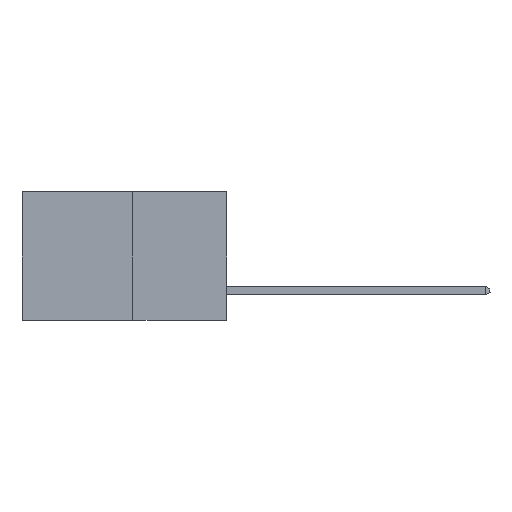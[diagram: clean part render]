
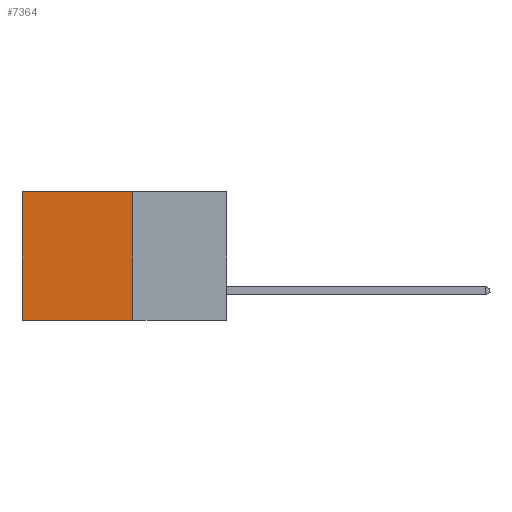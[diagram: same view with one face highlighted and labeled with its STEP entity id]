
A CAD part, left-side view. The second image highlights one B-rep face of the part: STEP entity #7364.
In plain terms, the highlighted planar face has unit normal (-1, 0, 0).
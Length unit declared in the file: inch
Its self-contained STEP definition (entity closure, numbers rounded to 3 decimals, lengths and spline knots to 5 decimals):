
#1385 = LINE ( 'NONE', #20983, #14818 ) ;
#3186 = CARTESIAN_POINT ( 'NONE',  ( 0.277, 0.59, -0.37 ) ) ;
#3329 = CARTESIAN_POINT ( 'NONE',  ( 0.277, 0.59, 0. ) ) ;
#3685 = EDGE_LOOP ( 'NONE', ( #13833, #16996, #8676, #19854 ) ) ;
#3715 = DIRECTION ( 'NONE',  ( 0., 0., -1. ) ) ;
#3744 = DIRECTION ( 'NONE',  ( 1., 0., 0. ) ) ;
#3790 = PLANE ( 'NONE',  #5228 ) ;
#3932 = VERTEX_POINT ( 'NONE', #3186 ) ;
#4126 = EDGE_CURVE ( 'NONE', #21635, #21733, #1385, .T. ) ;
#4231 = CARTESIAN_POINT ( 'NONE',  ( 0.277, 0.27, -0.37 ) ) ;
#5136 = LINE ( 'NONE', #8933, #22083 ) ;
#5228 = AXIS2_PLACEMENT_3D ( 'NONE', #4231, #3744, #3715 ) ;
#5536 = EDGE_CURVE ( 'NONE', #21733, #3932, #9169, .T. ) ;
#6329 = FACE_OUTER_BOUND ( 'NONE', #3685, .T. ) ;
#7364 = ADVANCED_FACE ( 'NONE', ( #6329 ), #3790, .F. ) ;
#8676 = ORIENTED_EDGE ( 'NONE', *, *, #4126, .F. ) ;
#8933 = CARTESIAN_POINT ( 'NONE',  ( 0.277, 0.59, -0.37 ) ) ;
#9169 = LINE ( 'NONE', #19328, #21474 ) ;
#9858 = CARTESIAN_POINT ( 'NONE',  ( 0.277, 0.27, -0.37 ) ) ;
#10268 = CARTESIAN_POINT ( 'NONE',  ( 0.277, 0.27, 0. ) ) ;
#10971 = VECTOR ( 'NONE', #15393, 39.37008 ) ;
#13833 = ORIENTED_EDGE ( 'NONE', *, *, #17235, .T. ) ;
#14818 = VECTOR ( 'NONE', #21877, 39.37008 ) ;
#15393 = DIRECTION ( 'NONE',  ( 0., 1., 0. ) ) ;
#15434 = EDGE_CURVE ( 'NONE', #21635, #21267, #19853, .T. ) ;
#15779 = DIRECTION ( 'NONE',  ( 0., 0., -1. ) ) ;
#16403 = CARTESIAN_POINT ( 'NONE',  ( 0.277, 0.27, 0. ) ) ;
#16996 = ORIENTED_EDGE ( 'NONE', *, *, #5536, .F. ) ;
#17235 = EDGE_CURVE ( 'NONE', #21267, #3932, #5136, .T. ) ;
#19238 = DIRECTION ( 'NONE',  ( 0., 1., 0. ) ) ;
#19328 = CARTESIAN_POINT ( 'NONE',  ( 0.277, 0.27, -0.37 ) ) ;
#19853 = LINE ( 'NONE', #10268, #10971 ) ;
#19854 = ORIENTED_EDGE ( 'NONE', *, *, #15434, .T. ) ;
#20983 = CARTESIAN_POINT ( 'NONE',  ( 0.277, 0.27, -0.37 ) ) ;
#21267 = VERTEX_POINT ( 'NONE', #3329 ) ;
#21474 = VECTOR ( 'NONE', #19238, 39.37008 ) ;
#21635 = VERTEX_POINT ( 'NONE', #16403 ) ;
#21733 = VERTEX_POINT ( 'NONE', #9858 ) ;
#21877 = DIRECTION ( 'NONE',  ( 0., 0., -1. ) ) ;
#22083 = VECTOR ( 'NONE', #15779, 39.37008 ) ;
